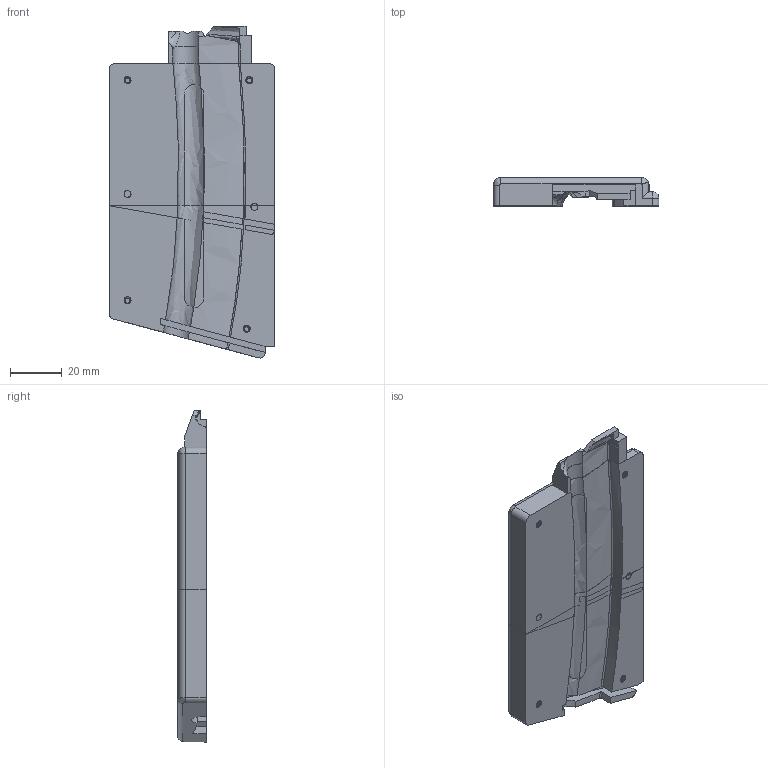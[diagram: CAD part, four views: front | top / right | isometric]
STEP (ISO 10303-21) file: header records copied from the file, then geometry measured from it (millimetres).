
FILE_DESCRIPTION(/* description */ (''),/* implementation_level */ '2;1');
FILE_NAME(/* name */ 'Right Body.step',/* time_stamp */ '2020-05-29T15:53:57-04:00',/* author */ (''),/* organization */ (''),/* preprocessor_version */ 'ST-DEVELOPER v18.1',/* originating_system */ 'Autodesk Translation Framework v9.3.0.1241',/* authorisation */ '');
FILE_SCHEMA (('AUTOMOTIVE_DESIGN { 1 0 10303 214 3 1 1 }'));
Products named in the file (3): Right Body; !; ! (1)
Assembly tree (2 placements, depth 2):
  Right Body
    !
    ! (1)
Bounding box: 64 x 11 x 128.15 mm (x, y, z)
Volume: 63050.3 mm3; surface area: 25939.4 mm2
Topology: 9 solids, 9 shells, 713 faces, 2050 edges, 1360 vertices
Faces by surface type: cylinder 406, bspline 205, plane 91, cone 10, sphere 1
Full cylindrical faces by diameter (mm): 2.35 x102, 3 x102
Entity records: 180031 total; most frequent: CARTESIAN_POINT 164328, ORIENTED_EDGE 4100, EDGE_CURVE 2050, DIRECTION 1999, VERTEX_POINT 1360, B_SPLINE_CURVE_WITH_KNOTS 1196, LINE 719, VECTOR 719
